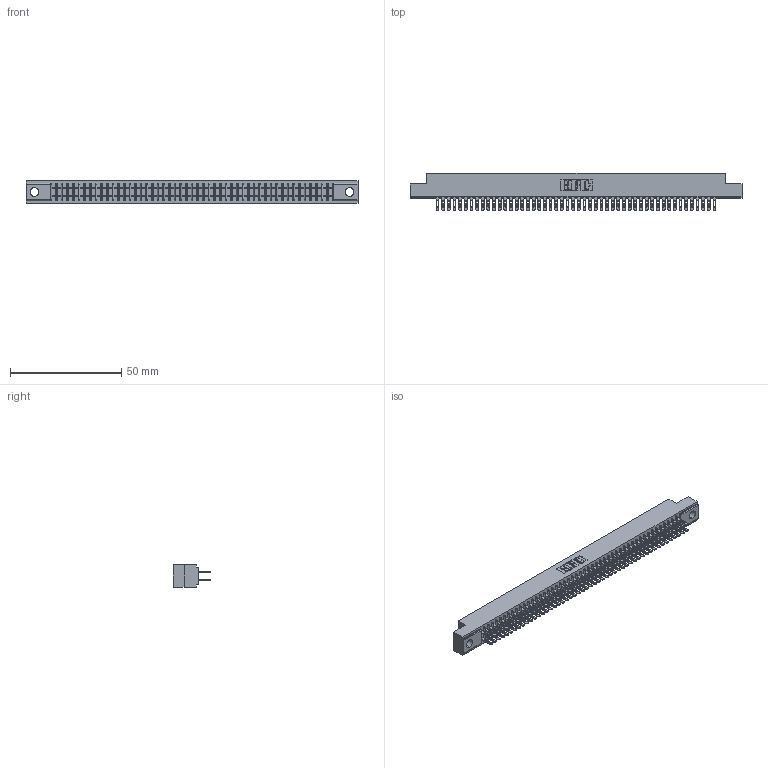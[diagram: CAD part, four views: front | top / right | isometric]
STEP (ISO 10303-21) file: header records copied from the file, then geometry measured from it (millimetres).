
FILE_DESCRIPTION (( 'STEP AP203' ), '1' );
FILE_NAME ('341-100-500-204.STEP', '2018-08-08T02:36:01', ( '' ), ( '' ), 'SwSTEP 2.0', 'SolidWorks 2016', '' );
FILE_SCHEMA (( 'CONFIG_CONTROL_DESIGN' ));
Products named in the file (3): 341-292-001_341-292-100; 341-100-500-204; 341 Part_.156 (3.96) Dia Mounting Holes
Assembly tree (101 placements, depth 2):
  341-100-500-204
    341 Part_.156 (3.96) Dia Mounting Holes
    341-292-001_341-292-100  x100
Bounding box: 149.22 x 16.69 x 10.16 mm (x, y, z)
Volume: 11049.7 mm3; surface area: 20587.4 mm2
Topology: 101 solids, 101 shells, 6730 faces, 19502 edges, 12630 vertices
Faces by surface type: plane 3882, cylinder 2648, sphere 102, torus 98
Entity records: 59871 total; most frequent: CARTESIAN_POINT 9956, ORIENTED_EDGE 9892, DIRECTION 9652, EDGE_CURVE 4946, VECTOR 4008, LINE 4008, VERTEX_POINT 3126, AXIS2_PLACEMENT_3D 2822
